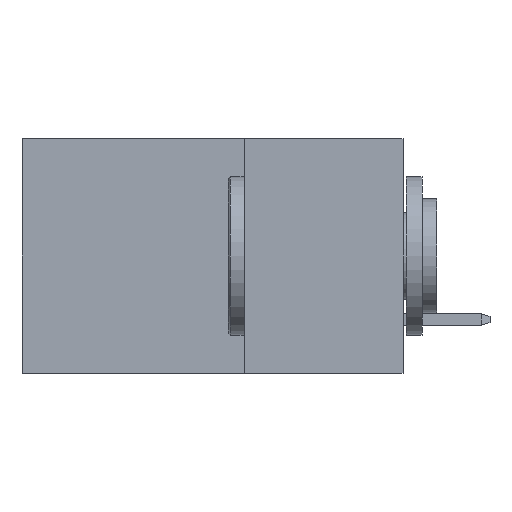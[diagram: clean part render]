
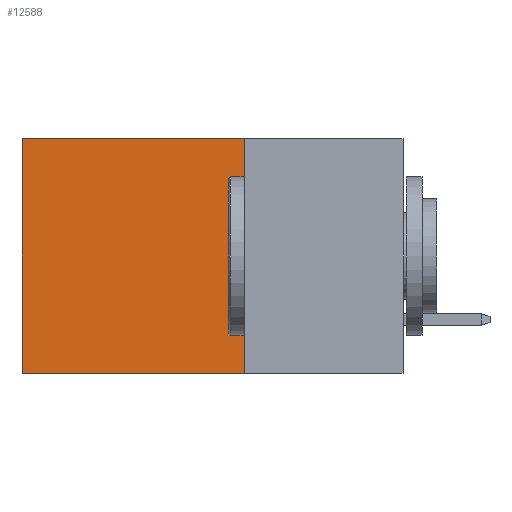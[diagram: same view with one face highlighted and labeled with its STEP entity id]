
A CAD part, left-side view. The second image highlights one B-rep face of the part: STEP entity #12588.
In plain terms, the highlighted planar face has unit normal (-1, 0, 0).
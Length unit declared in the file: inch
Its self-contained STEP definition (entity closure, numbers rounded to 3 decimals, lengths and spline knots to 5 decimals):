
#87 = DIRECTION ( 'NONE',  ( 0., 0., -1. ) ) ;
#154 = CARTESIAN_POINT ( 'NONE',  ( 0.2875, 0.25, 0. ) ) ;
#326 = ORIENTED_EDGE ( 'NONE', *, *, #4999, .F. ) ;
#475 = AXIS2_PLACEMENT_3D ( 'NONE', #8347, #8193, #87 ) ;
#1128 = PLANE ( 'NONE',  #475 ) ;
#1377 = ORIENTED_EDGE ( 'NONE', *, *, #3003, .F. ) ;
#1695 = CARTESIAN_POINT ( 'NONE',  ( 0.2875, 0.25, 0. ) ) ;
#2171 = CARTESIAN_POINT ( 'NONE',  ( 0.2875, 0.6, 0. ) ) ;
#2450 = EDGE_CURVE ( 'NONE', #4813, #8853, #4988, .T. ) ;
#2508 = ORIENTED_EDGE ( 'NONE', *, *, #8553, .T. ) ;
#2886 = VECTOR ( 'NONE', #12409, 39.37008 ) ;
#3003 = EDGE_CURVE ( 'NONE', #4813, #4135, #8761, .T. ) ;
#3267 = CARTESIAN_POINT ( 'NONE',  ( 0.2875, 0.6, -0.37 ) ) ;
#3537 = CARTESIAN_POINT ( 'NONE',  ( 0.2875, 0.25, -0.37 ) ) ;
#4135 = VERTEX_POINT ( 'NONE', #9421 ) ;
#4813 = VERTEX_POINT ( 'NONE', #154 ) ;
#4988 = LINE ( 'NONE', #6091, #2886 ) ;
#4999 = EDGE_CURVE ( 'NONE', #4135, #5922, #5772, .T. ) ;
#5637 = VECTOR ( 'NONE', #12390, 39.37008 ) ;
#5772 = LINE ( 'NONE', #3537, #9212 ) ;
#5922 = VERTEX_POINT ( 'NONE', #3267 ) ;
#6091 = CARTESIAN_POINT ( 'NONE',  ( 0.2875, 0.25, 0. ) ) ;
#7576 = DIRECTION ( 'NONE',  ( 0., 0., -1. ) ) ;
#8193 = DIRECTION ( 'NONE',  ( 1., 0., 0. ) ) ;
#8347 = CARTESIAN_POINT ( 'NONE',  ( 0.2875, 0.25, 0. ) ) ;
#8453 = ORIENTED_EDGE ( 'NONE', *, *, #2450, .T. ) ;
#8553 = EDGE_CURVE ( 'NONE', #8853, #5922, #12241, .T. ) ;
#8761 = LINE ( 'NONE', #1695, #5637 ) ;
#8853 = VERTEX_POINT ( 'NONE', #2171 ) ;
#9212 = VECTOR ( 'NONE', #14315, 39.37008 ) ;
#9421 = CARTESIAN_POINT ( 'NONE',  ( 0.2875, 0.25, -0.37 ) ) ;
#9531 = FACE_OUTER_BOUND ( 'NONE', #10286, .T. ) ;
#9944 = CARTESIAN_POINT ( 'NONE',  ( 0.2875, 0.6, 0. ) ) ;
#10286 = EDGE_LOOP ( 'NONE', ( #2508, #326, #1377, #8453 ) ) ;
#10524 = VECTOR ( 'NONE', #7576, 39.37008 ) ;
#12241 = LINE ( 'NONE', #9944, #10524 ) ;
#12390 = DIRECTION ( 'NONE',  ( 0., 0., -1. ) ) ;
#12409 = DIRECTION ( 'NONE',  ( 0., 1., 0. ) ) ;
#12588 = ADVANCED_FACE ( 'NONE', ( #9531 ), #1128, .F. ) ;
#14315 = DIRECTION ( 'NONE',  ( 0., 1., 0. ) ) ;
